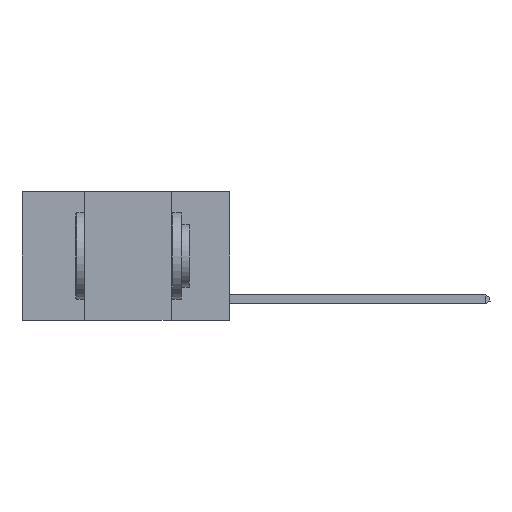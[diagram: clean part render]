
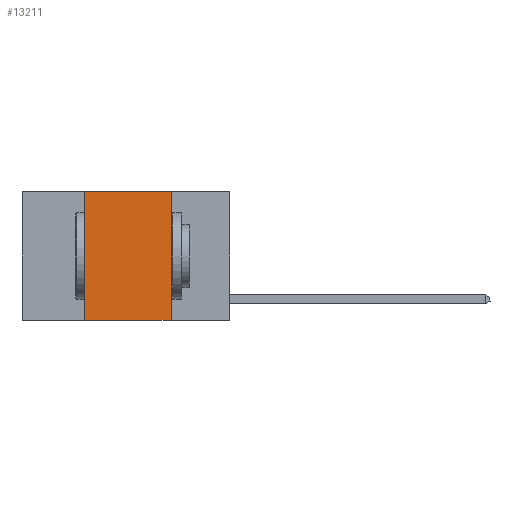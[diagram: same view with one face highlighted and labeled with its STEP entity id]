
A CAD part, left-side view. The second image highlights one B-rep face of the part: STEP entity #13211.
In plain terms, the highlighted planar face has unit normal (-1, 0, 0).
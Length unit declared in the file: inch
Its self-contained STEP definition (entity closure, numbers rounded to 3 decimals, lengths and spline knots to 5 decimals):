
#116 = EDGE_CURVE ( 'NONE', #7113, #18446, #1318, .T. ) ;
#309 = CARTESIAN_POINT ( 'NONE',  ( 0., 0.6, 0. ) ) ;
#1318 = LINE ( 'NONE', #16846, #1820 ) ;
#1574 = DIRECTION ( 'NONE',  ( 0., -1., 0. ) ) ;
#1820 = VECTOR ( 'NONE', #6695, 39.37008 ) ;
#1883 = DIRECTION ( 'NONE',  ( 0., -1., 0. ) ) ;
#1919 = DIRECTION ( 'NONE',  ( 0., 0., -1. ) ) ;
#3033 = CARTESIAN_POINT ( 'NONE',  ( 0., 0.17, 0. ) ) ;
#4590 = DIRECTION ( 'NONE',  ( 0., 0., 1. ) ) ;
#5150 = PLANE ( 'NONE',  #15862 ) ;
#5480 = EDGE_CURVE ( 'NONE', #15214, #8391, #18483, .T. ) ;
#6052 = VECTOR ( 'NONE', #4590, 39.37008 ) ;
#6695 = DIRECTION ( 'NONE',  ( 0., 0., -1. ) ) ;
#7113 = VERTEX_POINT ( 'NONE', #3033 ) ;
#7506 = VECTOR ( 'NONE', #1883, 39.37008 ) ;
#7839 = FACE_OUTER_BOUND ( 'NONE', #9526, .T. ) ;
#8093 = CARTESIAN_POINT ( 'NONE',  ( 0., 0.6, 0. ) ) ;
#8391 = VERTEX_POINT ( 'NONE', #19179 ) ;
#8811 = ORIENTED_EDGE ( 'NONE', *, *, #5480, .F. ) ;
#9136 = EDGE_CURVE ( 'NONE', #15214, #18446, #20487, .T. ) ;
#9526 = EDGE_LOOP ( 'NONE', ( #12132, #16449, #8811, #17480 ) ) ;
#10411 = VECTOR ( 'NONE', #1574, 39.37008 ) ;
#10919 = LINE ( 'NONE', #8093, #10411 ) ;
#11679 = DIRECTION ( 'NONE',  ( 1., 0., 0. ) ) ;
#12105 = CARTESIAN_POINT ( 'NONE',  ( 0., 0.42, -0.37 ) ) ;
#12132 = ORIENTED_EDGE ( 'NONE', *, *, #116, .F. ) ;
#12858 = CARTESIAN_POINT ( 'NONE',  ( 0., 0.17, -0.37 ) ) ;
#13211 = ADVANCED_FACE ( 'NONE', ( #7839 ), #5150, .F. ) ;
#13288 = CARTESIAN_POINT ( 'NONE',  ( 0., 0.6, -0.37 ) ) ;
#13757 = EDGE_CURVE ( 'NONE', #8391, #7113, #10919, .T. ) ;
#14315 = CARTESIAN_POINT ( 'NONE',  ( 0., 0.42, 0. ) ) ;
#15214 = VERTEX_POINT ( 'NONE', #12105 ) ;
#15862 = AXIS2_PLACEMENT_3D ( 'NONE', #309, #11679, #1919 ) ;
#16449 = ORIENTED_EDGE ( 'NONE', *, *, #13757, .F. ) ;
#16846 = CARTESIAN_POINT ( 'NONE',  ( 0., 0.17, 0. ) ) ;
#17480 = ORIENTED_EDGE ( 'NONE', *, *, #9136, .T. ) ;
#18446 = VERTEX_POINT ( 'NONE', #12858 ) ;
#18483 = LINE ( 'NONE', #14315, #6052 ) ;
#19179 = CARTESIAN_POINT ( 'NONE',  ( 0., 0.42, 0. ) ) ;
#20487 = LINE ( 'NONE', #13288, #7506 ) ;
